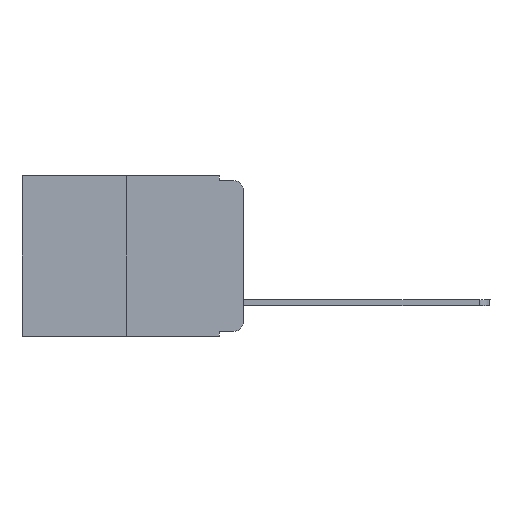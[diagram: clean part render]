
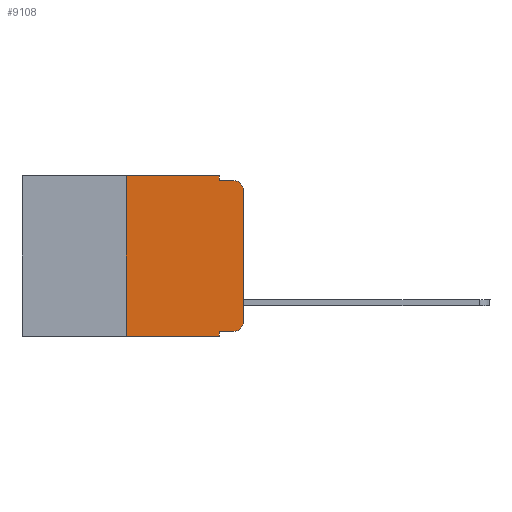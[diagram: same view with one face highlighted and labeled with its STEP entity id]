
A CAD part, left-side view. The second image highlights one B-rep face of the part: STEP entity #9108.
In plain terms, the highlighted planar face has unit normal (-1, 0, 0).
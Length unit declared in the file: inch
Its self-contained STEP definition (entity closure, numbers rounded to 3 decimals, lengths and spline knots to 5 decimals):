
#162 = VECTOR ( 'NONE', #4999, 39.37008 ) ;
#384 = CARTESIAN_POINT ( 'NONE',  ( 0., 0.051, 0. ) ) ;
#448 = CARTESIAN_POINT ( 'NONE',  ( 0., 0., -0.03 ) ) ;
#587 = DIRECTION ( 'NONE',  ( 0., 0., -1. ) ) ;
#726 = EDGE_CURVE ( 'NONE', #5899, #5076, #4093, .T. ) ;
#750 = PLANE ( 'NONE',  #9065 ) ;
#1069 = EDGE_CURVE ( 'NONE', #1463, #5834, #2292, .T. ) ;
#1142 = ORIENTED_EDGE ( 'NONE', *, *, #4509, .T. ) ;
#1204 = ORIENTED_EDGE ( 'NONE', *, *, #5185, .F. ) ;
#1346 = CARTESIAN_POINT ( 'NONE',  ( 0., 0., 0. ) ) ;
#1401 = VECTOR ( 'NONE', #4560, 39.37008 ) ;
#1410 = VERTEX_POINT ( 'NONE', #4173 ) ;
#1463 = VERTEX_POINT ( 'NONE', #2821 ) ;
#1529 = ORIENTED_EDGE ( 'NONE', *, *, #3494, .F. ) ;
#1621 = EDGE_LOOP ( 'NONE', ( #1142, #6269, #1204, #1529, #8514, #3897, #4791, #4823, #9565, #2854 ) ) ;
#1678 = LINE ( 'NONE', #6449, #6657 ) ;
#1695 = DIRECTION ( 'NONE',  ( 1., 0., 0. ) ) ;
#1787 = LINE ( 'NONE', #4942, #2537 ) ;
#1855 = LINE ( 'NONE', #8904, #162 ) ;
#2292 = CIRCLE ( 'NONE', #3763, 0.02 ) ;
#2537 = VECTOR ( 'NONE', #8152, 39.37008 ) ;
#2821 = CARTESIAN_POINT ( 'NONE',  ( 0., 0.02, -0.333 ) ) ;
#2854 = ORIENTED_EDGE ( 'NONE', *, *, #1069, .T. ) ;
#2891 = LINE ( 'NONE', #10153, #7219 ) ;
#2918 = AXIS2_PLACEMENT_3D ( 'NONE', #4657, #7026, #3041 ) ;
#2968 = CARTESIAN_POINT ( 'NONE',  ( 0., 0.051, 0. ) ) ;
#3041 = DIRECTION ( 'NONE',  ( 0., 0., -1. ) ) ;
#3105 = VERTEX_POINT ( 'NONE', #8241 ) ;
#3161 = CARTESIAN_POINT ( 'NONE',  ( 0., 0.25, -0.343 ) ) ;
#3192 = EDGE_CURVE ( 'NONE', #3105, #1463, #5277, .T. ) ;
#3494 = EDGE_CURVE ( 'NONE', #6851, #1410, #4138, .T. ) ;
#3763 = AXIS2_PLACEMENT_3D ( 'NONE', #5204, #8368, #9215 ) ;
#3897 = ORIENTED_EDGE ( 'NONE', *, *, #6439, .F. ) ;
#3918 = CARTESIAN_POINT ( 'NONE',  ( 0., 0.473, 0. ) ) ;
#4093 = CIRCLE ( 'NONE', #2918, 0.02 ) ;
#4138 = LINE ( 'NONE', #384, #7128 ) ;
#4173 = CARTESIAN_POINT ( 'NONE',  ( 0., 0.051, -0.01 ) ) ;
#4235 = CARTESIAN_POINT ( 'NONE',  ( 0., 0.051, -0.343 ) ) ;
#4369 = VERTEX_POINT ( 'NONE', #7417 ) ;
#4460 = EDGE_CURVE ( 'NONE', #5650, #5203, #6168, .T. ) ;
#4509 = EDGE_CURVE ( 'NONE', #5834, #5899, #6118, .T. ) ;
#4560 = DIRECTION ( 'NONE',  ( 0., 0., 1. ) ) ;
#4619 = CARTESIAN_POINT ( 'NONE',  ( 0., 0.473, -0.343 ) ) ;
#4657 = CARTESIAN_POINT ( 'NONE',  ( 0., 0.02, -0.03 ) ) ;
#4791 = ORIENTED_EDGE ( 'NONE', *, *, #4460, .T. ) ;
#4823 = ORIENTED_EDGE ( 'NONE', *, *, #4847, .F. ) ;
#4847 = EDGE_CURVE ( 'NONE', #3105, #5203, #2891, .T. ) ;
#4942 = CARTESIAN_POINT ( 'NONE',  ( 0., 0.25, 0. ) ) ;
#4999 = DIRECTION ( 'NONE',  ( 0., -1., 0. ) ) ;
#5076 = VERTEX_POINT ( 'NONE', #6316 ) ;
#5185 = EDGE_CURVE ( 'NONE', #1410, #5076, #1855, .T. ) ;
#5203 = VERTEX_POINT ( 'NONE', #4235 ) ;
#5204 = CARTESIAN_POINT ( 'NONE',  ( 0., 0.02, -0.313 ) ) ;
#5234 = EDGE_CURVE ( 'NONE', #4369, #6851, #1678, .T. ) ;
#5277 = LINE ( 'NONE', #6887, #9358 ) ;
#5650 = VERTEX_POINT ( 'NONE', #3161 ) ;
#5834 = VERTEX_POINT ( 'NONE', #9903 ) ;
#5899 = VERTEX_POINT ( 'NONE', #448 ) ;
#6118 = LINE ( 'NONE', #1346, #1401 ) ;
#6168 = LINE ( 'NONE', #4619, #8022 ) ;
#6269 = ORIENTED_EDGE ( 'NONE', *, *, #726, .T. ) ;
#6316 = CARTESIAN_POINT ( 'NONE',  ( 0., 0.02, -0.01 ) ) ;
#6362 = FACE_OUTER_BOUND ( 'NONE', #1621, .T. ) ;
#6439 = EDGE_CURVE ( 'NONE', #5650, #4369, #1787, .T. ) ;
#6449 = CARTESIAN_POINT ( 'NONE',  ( 0., 0.473, 0. ) ) ;
#6657 = VECTOR ( 'NONE', #8834, 39.37008 ) ;
#6851 = VERTEX_POINT ( 'NONE', #2968 ) ;
#6887 = CARTESIAN_POINT ( 'NONE',  ( 0., 0.051, -0.333 ) ) ;
#7026 = DIRECTION ( 'NONE',  ( -1., 0., 0. ) ) ;
#7081 = DIRECTION ( 'NONE',  ( 0., 0., -1. ) ) ;
#7128 = VECTOR ( 'NONE', #8223, 39.37008 ) ;
#7219 = VECTOR ( 'NONE', #587, 39.37008 ) ;
#7417 = CARTESIAN_POINT ( 'NONE',  ( 0., 0.25, 0. ) ) ;
#7771 = DIRECTION ( 'NONE',  ( 0., -1., 0. ) ) ;
#8022 = VECTOR ( 'NONE', #7771, 39.37008 ) ;
#8152 = DIRECTION ( 'NONE',  ( 0., 0., 1. ) ) ;
#8223 = DIRECTION ( 'NONE',  ( 0., 0., -1. ) ) ;
#8241 = CARTESIAN_POINT ( 'NONE',  ( 0., 0.051, -0.333 ) ) ;
#8344 = DIRECTION ( 'NONE',  ( 0., -1., 0. ) ) ;
#8368 = DIRECTION ( 'NONE',  ( -1., 0., 0. ) ) ;
#8514 = ORIENTED_EDGE ( 'NONE', *, *, #5234, .F. ) ;
#8834 = DIRECTION ( 'NONE',  ( 0., -1., 0. ) ) ;
#8904 = CARTESIAN_POINT ( 'NONE',  ( 0., 0.051, -0.01 ) ) ;
#9065 = AXIS2_PLACEMENT_3D ( 'NONE', #3918, #1695, #7081 ) ;
#9108 = ADVANCED_FACE ( 'NONE', ( #6362 ), #750, .F. ) ;
#9215 = DIRECTION ( 'NONE',  ( 0., 0., -1. ) ) ;
#9358 = VECTOR ( 'NONE', #8344, 39.37008 ) ;
#9565 = ORIENTED_EDGE ( 'NONE', *, *, #3192, .T. ) ;
#9903 = CARTESIAN_POINT ( 'NONE',  ( 0., 0., -0.313 ) ) ;
#10153 = CARTESIAN_POINT ( 'NONE',  ( 0., 0.051, 0. ) ) ;
